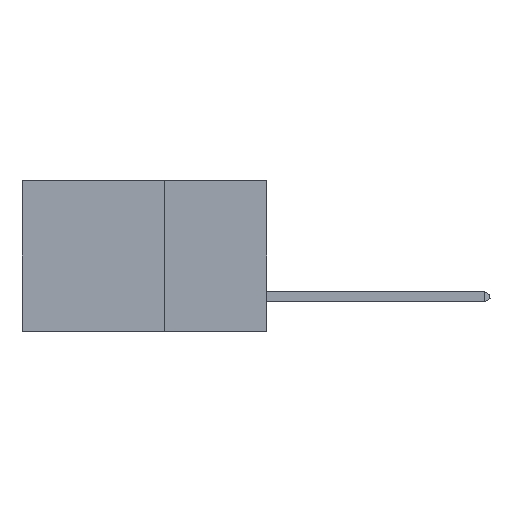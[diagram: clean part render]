
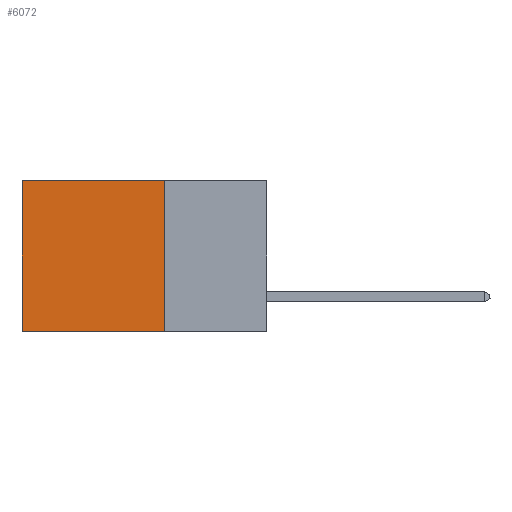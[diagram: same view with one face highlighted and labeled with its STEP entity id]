
A CAD part, left-side view. The second image highlights one B-rep face of the part: STEP entity #6072.
In plain terms, the highlighted planar face has unit normal (-1, 0, 0).
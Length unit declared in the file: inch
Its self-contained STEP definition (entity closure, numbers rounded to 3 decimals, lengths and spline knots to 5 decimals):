
#355 = EDGE_CURVE ( 'NONE', #2109, #24150, #19628, .T. ) ;
#1473 = CARTESIAN_POINT ( 'NONE',  ( 0.2875, 0.25, 0. ) ) ;
#1732 = CARTESIAN_POINT ( 'NONE',  ( 0.2875, 0.25, -0.37 ) ) ;
#2109 = VERTEX_POINT ( 'NONE', #17127 ) ;
#2319 = AXIS2_PLACEMENT_3D ( 'NONE', #1473, #15405, #35335 ) ;
#3461 = ORIENTED_EDGE ( 'NONE', *, *, #30817, .F. ) ;
#5546 = CARTESIAN_POINT ( 'NONE',  ( 0.2875, 0.25, 0. ) ) ;
#6072 = ADVANCED_FACE ( 'NONE', ( #32129 ), #32276, .F. ) ;
#6634 = VECTOR ( 'NONE', #10448, 39.37008 ) ;
#6693 = CARTESIAN_POINT ( 'NONE',  ( 0.2875, 0.25, 0. ) ) ;
#7103 = ORIENTED_EDGE ( 'NONE', *, *, #355, .T. ) ;
#7524 = EDGE_CURVE ( 'NONE', #14899, #14949, #10040, .T. ) ;
#7726 = EDGE_LOOP ( 'NONE', ( #7103, #3461, #18097, #23292 ) ) ;
#8540 = LINE ( 'NONE', #6693, #15624 ) ;
#10040 = LINE ( 'NONE', #19535, #17126 ) ;
#10448 = DIRECTION ( 'NONE',  ( 0., 1., 0. ) ) ;
#14899 = VERTEX_POINT ( 'NONE', #5546 ) ;
#14909 = CARTESIAN_POINT ( 'NONE',  ( 0.2875, 0.6, 0. ) ) ;
#14949 = VERTEX_POINT ( 'NONE', #17026 ) ;
#15405 = DIRECTION ( 'NONE',  ( 1., 0., 0. ) ) ;
#15624 = VECTOR ( 'NONE', #17938, 39.37008 ) ;
#17026 = CARTESIAN_POINT ( 'NONE',  ( 0.2875, 0.25, -0.37 ) ) ;
#17126 = VECTOR ( 'NONE', #19880, 39.37008 ) ;
#17127 = CARTESIAN_POINT ( 'NONE',  ( 0.2875, 0.6, 0. ) ) ;
#17938 = DIRECTION ( 'NONE',  ( 0., 1., 0. ) ) ;
#18097 = ORIENTED_EDGE ( 'NONE', *, *, #7524, .F. ) ;
#19535 = CARTESIAN_POINT ( 'NONE',  ( 0.2875, 0.25, 0. ) ) ;
#19628 = LINE ( 'NONE', #14909, #22290 ) ;
#19880 = DIRECTION ( 'NONE',  ( 0., 0., -1. ) ) ;
#20302 = LINE ( 'NONE', #1732, #6634 ) ;
#20869 = EDGE_CURVE ( 'NONE', #14899, #2109, #8540, .T. ) ;
#22290 = VECTOR ( 'NONE', #23298, 39.37008 ) ;
#23292 = ORIENTED_EDGE ( 'NONE', *, *, #20869, .T. ) ;
#23298 = DIRECTION ( 'NONE',  ( 0., 0., -1. ) ) ;
#24150 = VERTEX_POINT ( 'NONE', #30938 ) ;
#30817 = EDGE_CURVE ( 'NONE', #14949, #24150, #20302, .T. ) ;
#30938 = CARTESIAN_POINT ( 'NONE',  ( 0.2875, 0.6, -0.37 ) ) ;
#32129 = FACE_OUTER_BOUND ( 'NONE', #7726, .T. ) ;
#32276 = PLANE ( 'NONE',  #2319 ) ;
#35335 = DIRECTION ( 'NONE',  ( 0., 0., -1. ) ) ;
